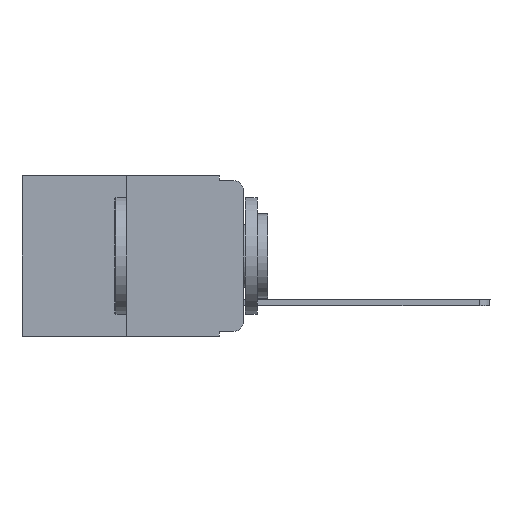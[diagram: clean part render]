
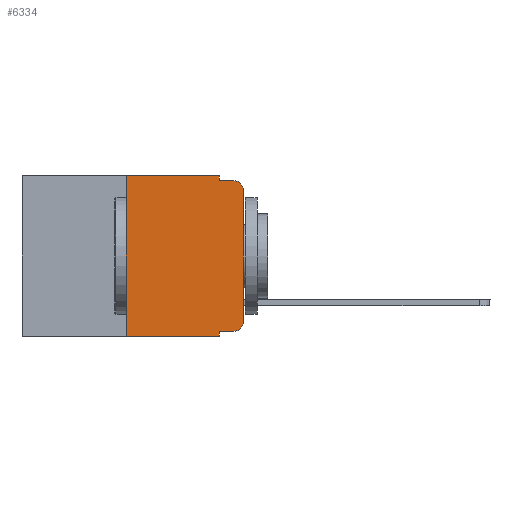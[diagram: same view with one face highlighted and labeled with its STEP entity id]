
A CAD part, left-side view. The second image highlights one B-rep face of the part: STEP entity #6334.
In plain terms, the highlighted planar face has unit normal (-1, 0, 0).
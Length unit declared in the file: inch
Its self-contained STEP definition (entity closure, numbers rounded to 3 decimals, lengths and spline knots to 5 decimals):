
#8 = LINE ( 'NONE', #8951, #7309 ) ;
#31 = VECTOR ( 'NONE', #1113, 39.37008 ) ;
#40 = VERTEX_POINT ( 'NONE', #6391 ) ;
#234 = ORIENTED_EDGE ( 'NONE', *, *, #7526, .T. ) ;
#632 = EDGE_CURVE ( 'NONE', #3261, #4006, #5161, .T. ) ;
#668 = VECTOR ( 'NONE', #6343, 39.37008 ) ;
#779 = CARTESIAN_POINT ( 'NONE',  ( 0., 0.051, -0.333 ) ) ;
#783 = DIRECTION ( 'NONE',  ( 1., 0., 0. ) ) ;
#957 = LINE ( 'NONE', #9481, #6477 ) ;
#1108 = CARTESIAN_POINT ( 'NONE',  ( 0., 0.473, -0.343 ) ) ;
#1113 = DIRECTION ( 'NONE',  ( 0., -1., 0. ) ) ;
#1288 = ORIENTED_EDGE ( 'NONE', *, *, #632, .F. ) ;
#1326 = DIRECTION ( 'NONE',  ( 0., 0., -1. ) ) ;
#1527 = CIRCLE ( 'NONE', #8593, 0.02 ) ;
#1748 = DIRECTION ( 'NONE',  ( 0., 0., -1. ) ) ;
#1766 = EDGE_CURVE ( 'NONE', #6423, #3510, #4952, .T. ) ;
#2047 = CARTESIAN_POINT ( 'NONE',  ( 0., 0.02, -0.03 ) ) ;
#2239 = ORIENTED_EDGE ( 'NONE', *, *, #4390, .F. ) ;
#2377 = DIRECTION ( 'NONE',  ( 0., 0., -1. ) ) ;
#2429 = CARTESIAN_POINT ( 'NONE',  ( 0., 0.25, -0.343 ) ) ;
#2503 = CARTESIAN_POINT ( 'NONE',  ( 0., 0.051, 0. ) ) ;
#2551 = VECTOR ( 'NONE', #1748, 39.37008 ) ;
#2695 = LINE ( 'NONE', #7085, #5400 ) ;
#2786 = CARTESIAN_POINT ( 'NONE',  ( 0., 0., -0.03 ) ) ;
#2897 = CARTESIAN_POINT ( 'NONE',  ( 0., 0.473, 0. ) ) ;
#2944 = EDGE_CURVE ( 'NONE', #8119, #40, #4662, .T. ) ;
#3149 = ORIENTED_EDGE ( 'NONE', *, *, #4733, .T. ) ;
#3173 = DIRECTION ( 'NONE',  ( 0., 0., 1. ) ) ;
#3261 = VERTEX_POINT ( 'NONE', #9189 ) ;
#3510 = VERTEX_POINT ( 'NONE', #7725 ) ;
#3613 = VERTEX_POINT ( 'NONE', #3825 ) ;
#3767 = ORIENTED_EDGE ( 'NONE', *, *, #1766, .F. ) ;
#3825 = CARTESIAN_POINT ( 'NONE',  ( 0., 0.051, -0.343 ) ) ;
#3885 = VERTEX_POINT ( 'NONE', #2429 ) ;
#3904 = ORIENTED_EDGE ( 'NONE', *, *, #4180, .F. ) ;
#3974 = CARTESIAN_POINT ( 'NONE',  ( 0., 0., -0.313 ) ) ;
#4006 = VERTEX_POINT ( 'NONE', #5913 ) ;
#4180 = EDGE_CURVE ( 'NONE', #3510, #3261, #2695, .T. ) ;
#4390 = EDGE_CURVE ( 'NONE', #8119, #3613, #6136, .T. ) ;
#4483 = DIRECTION ( 'NONE',  ( 0., -1., 0. ) ) ;
#4612 = LINE ( 'NONE', #1108, #5261 ) ;
#4643 = FACE_OUTER_BOUND ( 'NONE', #7313, .T. ) ;
#4662 = LINE ( 'NONE', #6227, #668 ) ;
#4733 = EDGE_CURVE ( 'NONE', #3885, #3613, #4612, .T. ) ;
#4862 = ORIENTED_EDGE ( 'NONE', *, *, #6272, .T. ) ;
#4952 = LINE ( 'NONE', #2897, #31 ) ;
#5161 = LINE ( 'NONE', #10177, #5914 ) ;
#5261 = VECTOR ( 'NONE', #9253, 39.37008 ) ;
#5400 = VECTOR ( 'NONE', #8784, 39.37008 ) ;
#5706 = CARTESIAN_POINT ( 'NONE',  ( 0., 0.473, 0. ) ) ;
#5913 = CARTESIAN_POINT ( 'NONE',  ( 0., 0.02, -0.01 ) ) ;
#5914 = VECTOR ( 'NONE', #4483, 39.37008 ) ;
#6136 = LINE ( 'NONE', #2503, #2551 ) ;
#6227 = CARTESIAN_POINT ( 'NONE',  ( 0., 0.051, -0.333 ) ) ;
#6232 = DIRECTION ( 'NONE',  ( -1., 0., 0. ) ) ;
#6272 = EDGE_CURVE ( 'NONE', #6845, #10238, #8, .T. ) ;
#6321 = ORIENTED_EDGE ( 'NONE', *, *, #8540, .T. ) ;
#6334 = ADVANCED_FACE ( 'NONE', ( #4643 ), #6466, .F. ) ;
#6343 = DIRECTION ( 'NONE',  ( 0., -1., 0. ) ) ;
#6383 = CIRCLE ( 'NONE', #9460, 0.02 ) ;
#6391 = CARTESIAN_POINT ( 'NONE',  ( 0., 0.02, -0.333 ) ) ;
#6423 = VERTEX_POINT ( 'NONE', #9097 ) ;
#6466 = PLANE ( 'NONE',  #9487 ) ;
#6477 = VECTOR ( 'NONE', #6955, 39.37008 ) ;
#6505 = DIRECTION ( 'NONE',  ( -1., 0., 0. ) ) ;
#6845 = VERTEX_POINT ( 'NONE', #3974 ) ;
#6955 = DIRECTION ( 'NONE',  ( 0., 0., 1. ) ) ;
#7085 = CARTESIAN_POINT ( 'NONE',  ( 0., 0.051, 0. ) ) ;
#7210 = ORIENTED_EDGE ( 'NONE', *, *, #10414, .F. ) ;
#7309 = VECTOR ( 'NONE', #3173, 39.37008 ) ;
#7313 = EDGE_LOOP ( 'NONE', ( #4862, #6321, #1288, #3904, #3767, #7210, #3149, #2239, #9531, #234 ) ) ;
#7526 = EDGE_CURVE ( 'NONE', #40, #6845, #1527, .T. ) ;
#7725 = CARTESIAN_POINT ( 'NONE',  ( 0., 0.051, 0. ) ) ;
#8119 = VERTEX_POINT ( 'NONE', #779 ) ;
#8145 = DIRECTION ( 'NONE',  ( 0., 0., -1. ) ) ;
#8540 = EDGE_CURVE ( 'NONE', #10238, #4006, #6383, .T. ) ;
#8593 = AXIS2_PLACEMENT_3D ( 'NONE', #9675, #6505, #8145 ) ;
#8784 = DIRECTION ( 'NONE',  ( 0., 0., -1. ) ) ;
#8951 = CARTESIAN_POINT ( 'NONE',  ( 0., 0., 0. ) ) ;
#9097 = CARTESIAN_POINT ( 'NONE',  ( 0., 0.25, 0. ) ) ;
#9189 = CARTESIAN_POINT ( 'NONE',  ( 0., 0.051, -0.01 ) ) ;
#9253 = DIRECTION ( 'NONE',  ( 0., -1., 0. ) ) ;
#9460 = AXIS2_PLACEMENT_3D ( 'NONE', #2047, #6232, #1326 ) ;
#9481 = CARTESIAN_POINT ( 'NONE',  ( 0., 0.25, 0. ) ) ;
#9487 = AXIS2_PLACEMENT_3D ( 'NONE', #5706, #783, #2377 ) ;
#9531 = ORIENTED_EDGE ( 'NONE', *, *, #2944, .T. ) ;
#9675 = CARTESIAN_POINT ( 'NONE',  ( 0., 0.02, -0.313 ) ) ;
#10177 = CARTESIAN_POINT ( 'NONE',  ( 0., 0.051, -0.01 ) ) ;
#10238 = VERTEX_POINT ( 'NONE', #2786 ) ;
#10414 = EDGE_CURVE ( 'NONE', #3885, #6423, #957, .T. ) ;
